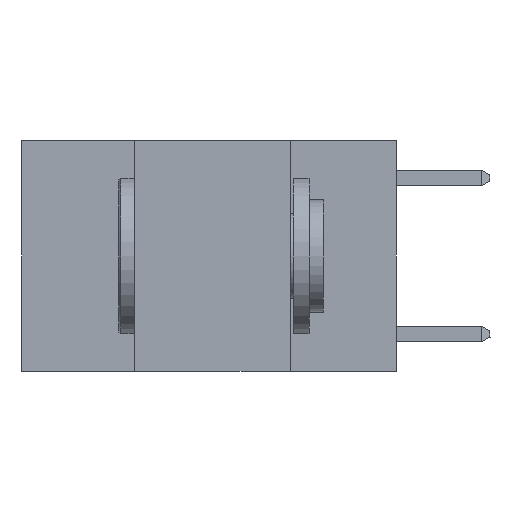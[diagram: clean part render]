
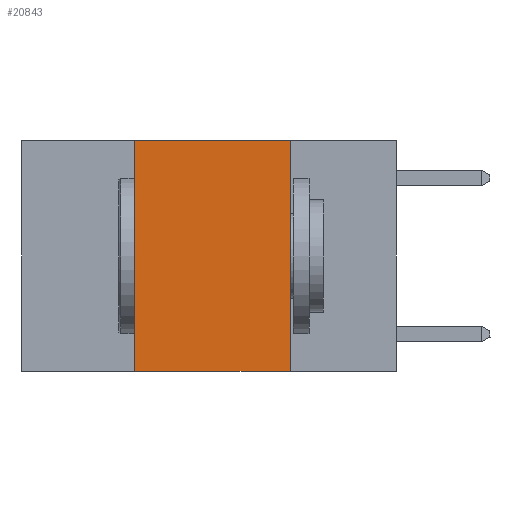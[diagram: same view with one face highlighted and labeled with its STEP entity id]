
A CAD part, left-side view. The second image highlights one B-rep face of the part: STEP entity #20843.
In plain terms, the highlighted planar face has unit normal (-1, 0, 0).
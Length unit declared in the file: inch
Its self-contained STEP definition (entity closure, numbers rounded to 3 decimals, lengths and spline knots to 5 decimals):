
#110 = EDGE_CURVE ( 'NONE', #2626, #10091, #8456, .T. ) ;
#112 = EDGE_CURVE ( 'NONE', #16690, #463, #17148, .T. ) ;
#193 = EDGE_CURVE ( 'NONE', #2626, #463, #12084, .T. ) ;
#463 = VERTEX_POINT ( 'NONE', #1449 ) ;
#1105 = DIRECTION ( 'NONE',  ( 0., 0., 1. ) ) ;
#1449 = CARTESIAN_POINT ( 'NONE',  ( 0., 0.17, -0.37 ) ) ;
#1494 = LINE ( 'NONE', #4662, #6408 ) ;
#2626 = VERTEX_POINT ( 'NONE', #16673 ) ;
#4170 = AXIS2_PLACEMENT_3D ( 'NONE', #21635, #7749, #21713 ) ;
#4446 = CARTESIAN_POINT ( 'NONE',  ( 0., 0.17, 0. ) ) ;
#4662 = CARTESIAN_POINT ( 'NONE',  ( 0., 0.6, 0. ) ) ;
#6408 = VECTOR ( 'NONE', #22594, 39.37008 ) ;
#7175 = EDGE_LOOP ( 'NONE', ( #13597, #23964, #19574, #16800 ) ) ;
#7749 = DIRECTION ( 'NONE',  ( 1., 0., 0. ) ) ;
#8456 = LINE ( 'NONE', #8941, #8757 ) ;
#8742 = DIRECTION ( 'NONE',  ( 0., 0., -1. ) ) ;
#8757 = VECTOR ( 'NONE', #1105, 39.37008 ) ;
#8941 = CARTESIAN_POINT ( 'NONE',  ( 0., 0.42, 0. ) ) ;
#9034 = CARTESIAN_POINT ( 'NONE',  ( 0., 0.17, 0. ) ) ;
#10036 = CARTESIAN_POINT ( 'NONE',  ( 0., 0.42, 0. ) ) ;
#10091 = VERTEX_POINT ( 'NONE', #10036 ) ;
#10441 = CARTESIAN_POINT ( 'NONE',  ( 0., 0.6, -0.37 ) ) ;
#11697 = VECTOR ( 'NONE', #20189, 39.37008 ) ;
#12084 = LINE ( 'NONE', #10441, #11697 ) ;
#13597 = ORIENTED_EDGE ( 'NONE', *, *, #112, .F. ) ;
#13615 = EDGE_CURVE ( 'NONE', #10091, #16690, #1494, .T. ) ;
#15844 = PLANE ( 'NONE',  #4170 ) ;
#16673 = CARTESIAN_POINT ( 'NONE',  ( 0., 0.42, -0.37 ) ) ;
#16690 = VERTEX_POINT ( 'NONE', #4446 ) ;
#16800 = ORIENTED_EDGE ( 'NONE', *, *, #193, .T. ) ;
#17148 = LINE ( 'NONE', #9034, #19940 ) ;
#18823 = FACE_OUTER_BOUND ( 'NONE', #7175, .T. ) ;
#19574 = ORIENTED_EDGE ( 'NONE', *, *, #110, .F. ) ;
#19940 = VECTOR ( 'NONE', #8742, 39.37008 ) ;
#20189 = DIRECTION ( 'NONE',  ( 0., -1., 0. ) ) ;
#20843 = ADVANCED_FACE ( 'NONE', ( #18823 ), #15844, .F. ) ;
#21635 = CARTESIAN_POINT ( 'NONE',  ( 0., 0.6, 0. ) ) ;
#21713 = DIRECTION ( 'NONE',  ( 0., 0., -1. ) ) ;
#22594 = DIRECTION ( 'NONE',  ( 0., -1., 0. ) ) ;
#23964 = ORIENTED_EDGE ( 'NONE', *, *, #13615, .F. ) ;
